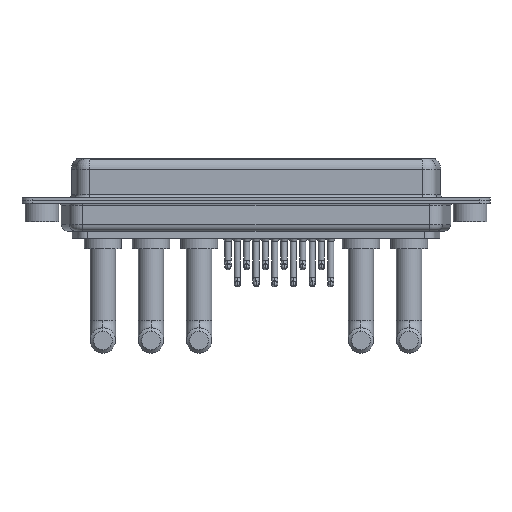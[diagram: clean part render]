
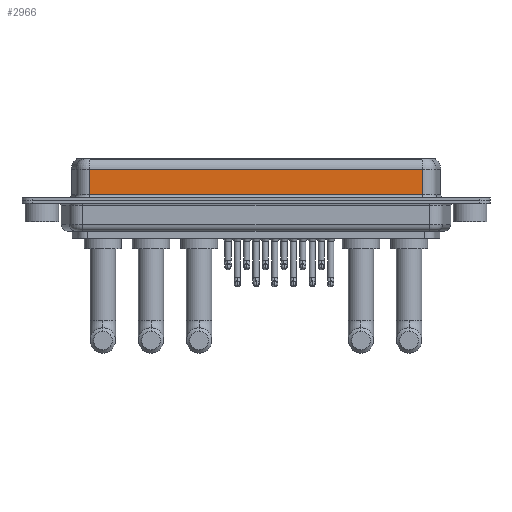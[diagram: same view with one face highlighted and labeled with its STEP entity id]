
A CAD part, front view. The second image highlights one B-rep face of the part: STEP entity #2966.
In plain terms, the highlighted planar face has unit normal (0, -1, 0).
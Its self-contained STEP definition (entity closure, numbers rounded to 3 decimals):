
#305 = CARTESIAN_POINT ( 'NONE',  ( 56.462, -3.95, 4.65 ) ) ;
#1152 = LINE ( 'NONE', #9242, #10726 ) ;
#2058 = VECTOR ( 'NONE', #17065, 1000. ) ;
#2409 = VERTEX_POINT ( 'NONE', #6738 ) ;
#2966 = ADVANCED_FACE ( 'NONE', ( #13580 ), #8862, .F. ) ;
#3949 = ORIENTED_EDGE ( 'NONE', *, *, #14646, .T. ) ;
#4389 = VERTEX_POINT ( 'NONE', #15322 ) ;
#4790 = VERTEX_POINT ( 'NONE', #16575 ) ;
#5195 = DIRECTION ( 'NONE',  ( 1., 0., 0. ) ) ;
#5197 = ORIENTED_EDGE ( 'NONE', *, *, #11878, .F. ) ;
#5494 = CARTESIAN_POINT ( 'NONE',  ( 56.462, -3.95, 6.4 ) ) ;
#6177 = LINE ( 'NONE', #305, #15911 ) ;
#6738 = CARTESIAN_POINT ( 'NONE',  ( 7.038, -3.95, 0.9 ) ) ;
#7415 = DIRECTION ( 'NONE',  ( 0., 0., -1. ) ) ;
#8862 = PLANE ( 'NONE',  #13421 ) ;
#9242 = CARTESIAN_POINT ( 'NONE',  ( 56.462, -3.95, 6.4 ) ) ;
#10726 = VECTOR ( 'NONE', #7415, 1000. ) ;
#11038 = LINE ( 'NONE', #18918, #11187 ) ;
#11187 = VECTOR ( 'NONE', #5195, 1000. ) ;
#11701 = ORIENTED_EDGE ( 'NONE', *, *, #11969, .T. ) ;
#11878 = EDGE_CURVE ( 'NONE', #16745, #4389, #1152, .T. ) ;
#11969 = EDGE_CURVE ( 'NONE', #16745, #4790, #6177, .T. ) ;
#12250 = LINE ( 'NONE', #15334, #2058 ) ;
#12612 = EDGE_LOOP ( 'NONE', ( #5197, #11701, #16095, #3949 ) ) ;
#12978 = CARTESIAN_POINT ( 'NONE',  ( 56.462, -3.95, 4.65 ) ) ;
#13421 = AXIS2_PLACEMENT_3D ( 'NONE', #5494, #19723, #15216 ) ;
#13580 = FACE_OUTER_BOUND ( 'NONE', #12612, .T. ) ;
#14646 = EDGE_CURVE ( 'NONE', #2409, #4389, #11038, .T. ) ;
#15216 = DIRECTION ( 'NONE',  ( 0., 0., 1. ) ) ;
#15322 = CARTESIAN_POINT ( 'NONE',  ( 56.462, -3.95, 0.9 ) ) ;
#15334 = CARTESIAN_POINT ( 'NONE',  ( 7.038, -3.95, 6.4 ) ) ;
#15911 = VECTOR ( 'NONE', #17535, 1000. ) ;
#16095 = ORIENTED_EDGE ( 'NONE', *, *, #17025, .T. ) ;
#16575 = CARTESIAN_POINT ( 'NONE',  ( 7.038, -3.95, 4.65 ) ) ;
#16745 = VERTEX_POINT ( 'NONE', #12978 ) ;
#17025 = EDGE_CURVE ( 'NONE', #4790, #2409, #12250, .T. ) ;
#17065 = DIRECTION ( 'NONE',  ( 0., 0., -1. ) ) ;
#17535 = DIRECTION ( 'NONE',  ( -1., 0., 0. ) ) ;
#18918 = CARTESIAN_POINT ( 'NONE',  ( 56.462, -3.95, 0.9 ) ) ;
#19723 = DIRECTION ( 'NONE',  ( 0., 1., 0. ) ) ;
